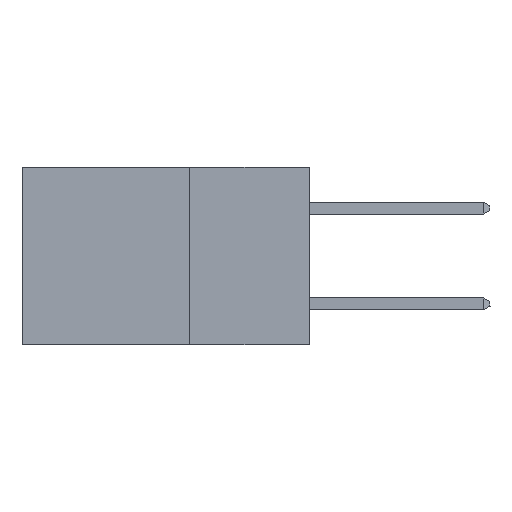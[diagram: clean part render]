
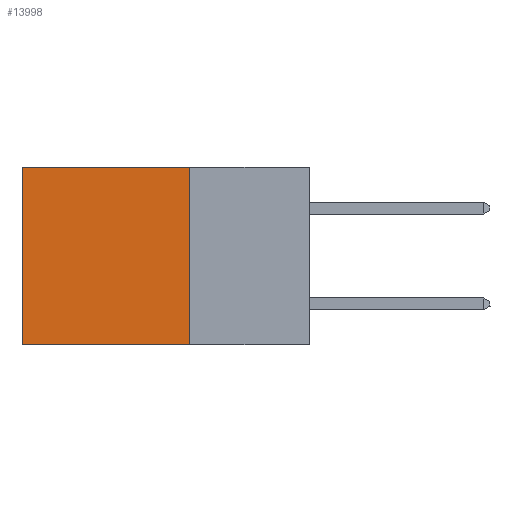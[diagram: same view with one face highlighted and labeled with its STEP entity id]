
A CAD part, left-side view. The second image highlights one B-rep face of the part: STEP entity #13998.
In plain terms, the highlighted planar face has unit normal (-1, 0, 0).
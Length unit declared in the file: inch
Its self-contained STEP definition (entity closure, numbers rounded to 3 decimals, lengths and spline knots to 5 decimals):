
#732 = VERTEX_POINT ( 'NONE', #29906 ) ;
#2464 = PLANE ( 'NONE',  #25549 ) ;
#3192 = EDGE_LOOP ( 'NONE', ( #3306, #14377, #9089, #3635 ) ) ;
#3306 = ORIENTED_EDGE ( 'NONE', *, *, #13221, .T. ) ;
#3635 = ORIENTED_EDGE ( 'NONE', *, *, #9948, .T. ) ;
#6598 = VECTOR ( 'NONE', #7476, 39.37008 ) ;
#7476 = DIRECTION ( 'NONE',  ( 0., 1., 0. ) ) ;
#7646 = LINE ( 'NONE', #19180, #29689 ) ;
#8451 = CARTESIAN_POINT ( 'NONE',  ( 0.2875, 0.25, 0. ) ) ;
#8651 = VECTOR ( 'NONE', #29228, 39.37008 ) ;
#9089 = ORIENTED_EDGE ( 'NONE', *, *, #16334, .F. ) ;
#9948 = EDGE_CURVE ( 'NONE', #35343, #732, #13986, .T. ) ;
#13221 = EDGE_CURVE ( 'NONE', #732, #22825, #7646, .T. ) ;
#13986 = LINE ( 'NONE', #34000, #34336 ) ;
#13998 = ADVANCED_FACE ( 'NONE', ( #28386 ), #2464, .F. ) ;
#14377 = ORIENTED_EDGE ( 'NONE', *, *, #30834, .F. ) ;
#16334 = EDGE_CURVE ( 'NONE', #35343, #18045, #17704, .T. ) ;
#16352 = DIRECTION ( 'NONE',  ( 0., 0., -1. ) ) ;
#17018 = DIRECTION ( 'NONE',  ( 0., 1., 0. ) ) ;
#17704 = LINE ( 'NONE', #8451, #8651 ) ;
#18045 = VERTEX_POINT ( 'NONE', #27513 ) ;
#19180 = CARTESIAN_POINT ( 'NONE',  ( 0.2875, 0.6, 0. ) ) ;
#19315 = CARTESIAN_POINT ( 'NONE',  ( 0.2875, 0.25, 0. ) ) ;
#22825 = VERTEX_POINT ( 'NONE', #35751 ) ;
#24121 = CARTESIAN_POINT ( 'NONE',  ( 0.2875, 0.25, -0.37 ) ) ;
#25549 = AXIS2_PLACEMENT_3D ( 'NONE', #19315, #36669, #33835 ) ;
#26424 = CARTESIAN_POINT ( 'NONE',  ( 0.2875, 0.25, 0. ) ) ;
#27513 = CARTESIAN_POINT ( 'NONE',  ( 0.2875, 0.25, -0.37 ) ) ;
#28386 = FACE_OUTER_BOUND ( 'NONE', #3192, .T. ) ;
#29228 = DIRECTION ( 'NONE',  ( 0., 0., -1. ) ) ;
#29689 = VECTOR ( 'NONE', #16352, 39.37008 ) ;
#29906 = CARTESIAN_POINT ( 'NONE',  ( 0.2875, 0.6, 0. ) ) ;
#30834 = EDGE_CURVE ( 'NONE', #18045, #22825, #33346, .T. ) ;
#33346 = LINE ( 'NONE', #24121, #6598 ) ;
#33835 = DIRECTION ( 'NONE',  ( 0., 0., -1. ) ) ;
#34000 = CARTESIAN_POINT ( 'NONE',  ( 0.2875, 0.25, 0. ) ) ;
#34336 = VECTOR ( 'NONE', #17018, 39.37008 ) ;
#35343 = VERTEX_POINT ( 'NONE', #26424 ) ;
#35751 = CARTESIAN_POINT ( 'NONE',  ( 0.2875, 0.6, -0.37 ) ) ;
#36669 = DIRECTION ( 'NONE',  ( 1., 0., 0. ) ) ;
